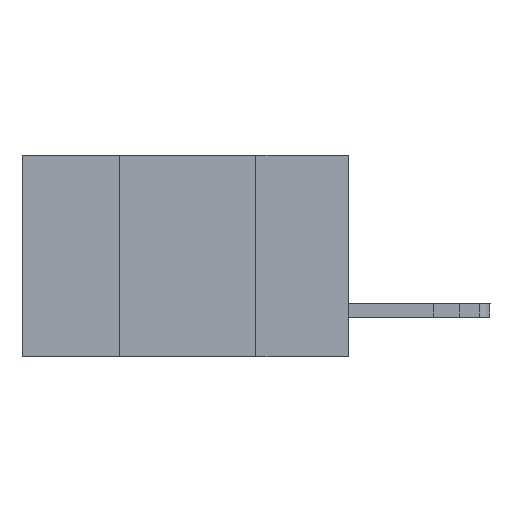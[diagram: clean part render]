
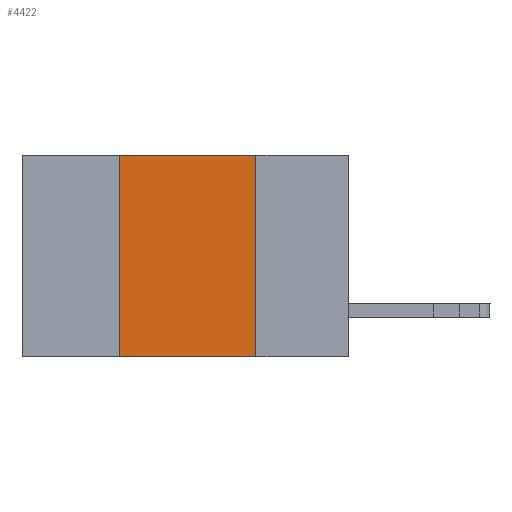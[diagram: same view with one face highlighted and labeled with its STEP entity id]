
A CAD part, left-side view. The second image highlights one B-rep face of the part: STEP entity #4422.
In plain terms, the highlighted planar face has unit normal (-1, 0, 0).
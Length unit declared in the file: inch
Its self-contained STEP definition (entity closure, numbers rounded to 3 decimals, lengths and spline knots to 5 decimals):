
#6 = EDGE_CURVE ( 'NONE', #8318, #7124, #7148, .T. ) ;
#78 = CARTESIAN_POINT ( 'NONE',  ( 0., 0.17, -0.37 ) ) ;
#225 = DIRECTION ( 'NONE',  ( 0., -1., 0. ) ) ;
#1756 = VECTOR ( 'NONE', #10436, 39.37008 ) ;
#1965 = VERTEX_POINT ( 'NONE', #4154 ) ;
#2511 = ORIENTED_EDGE ( 'NONE', *, *, #14212, .F. ) ;
#3142 = ORIENTED_EDGE ( 'NONE', *, *, #12361, .F. ) ;
#3385 = CARTESIAN_POINT ( 'NONE',  ( 0., 0.6, 0. ) ) ;
#3508 = CARTESIAN_POINT ( 'NONE',  ( 0., 0.6, 0. ) ) ;
#3584 = AXIS2_PLACEMENT_3D ( 'NONE', #3508, #8413, #8577 ) ;
#3769 = DIRECTION ( 'NONE',  ( 0., 0., -1. ) ) ;
#4024 = CARTESIAN_POINT ( 'NONE',  ( 0., 0.42, 0. ) ) ;
#4154 = CARTESIAN_POINT ( 'NONE',  ( 0., 0.17, -0.37 ) ) ;
#4219 = ORIENTED_EDGE ( 'NONE', *, *, #6, .F. ) ;
#4422 = ADVANCED_FACE ( 'NONE', ( #4880 ), #6000, .F. ) ;
#4880 = FACE_OUTER_BOUND ( 'NONE', #13480, .T. ) ;
#6000 = PLANE ( 'NONE',  #3584 ) ;
#6403 = LINE ( 'NONE', #11059, #15370 ) ;
#7124 = VERTEX_POINT ( 'NONE', #4024 ) ;
#7148 = LINE ( 'NONE', #13071, #13454 ) ;
#7323 = ORIENTED_EDGE ( 'NONE', *, *, #14877, .T. ) ;
#8285 = LINE ( 'NONE', #3385, #1756 ) ;
#8318 = VERTEX_POINT ( 'NONE', #15696 ) ;
#8413 = DIRECTION ( 'NONE',  ( 1., 0., 0. ) ) ;
#8577 = DIRECTION ( 'NONE',  ( 0., 0., -1. ) ) ;
#9232 = VECTOR ( 'NONE', #3769, 39.37008 ) ;
#9524 = CARTESIAN_POINT ( 'NONE',  ( 0., 0.17, 0. ) ) ;
#10436 = DIRECTION ( 'NONE',  ( 0., -1., 0. ) ) ;
#10509 = DIRECTION ( 'NONE',  ( 0., 0., 1. ) ) ;
#11059 = CARTESIAN_POINT ( 'NONE',  ( 0., 0.6, -0.37 ) ) ;
#11532 = VERTEX_POINT ( 'NONE', #9524 ) ;
#12361 = EDGE_CURVE ( 'NONE', #7124, #11532, #8285, .T. ) ;
#13071 = CARTESIAN_POINT ( 'NONE',  ( 0., 0.42, -0.37 ) ) ;
#13454 = VECTOR ( 'NONE', #10509, 39.37008 ) ;
#13480 = EDGE_LOOP ( 'NONE', ( #2511, #3142, #4219, #7323 ) ) ;
#14212 = EDGE_CURVE ( 'NONE', #11532, #1965, #15648, .T. ) ;
#14877 = EDGE_CURVE ( 'NONE', #8318, #1965, #6403, .T. ) ;
#15370 = VECTOR ( 'NONE', #225, 39.37008 ) ;
#15648 = LINE ( 'NONE', #78, #9232 ) ;
#15696 = CARTESIAN_POINT ( 'NONE',  ( 0., 0.42, -0.37 ) ) ;
